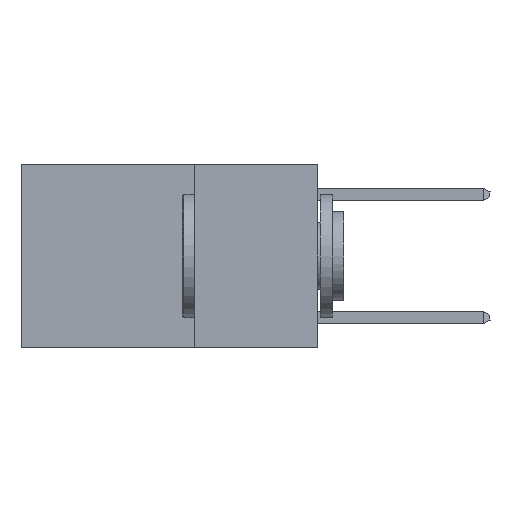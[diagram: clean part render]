
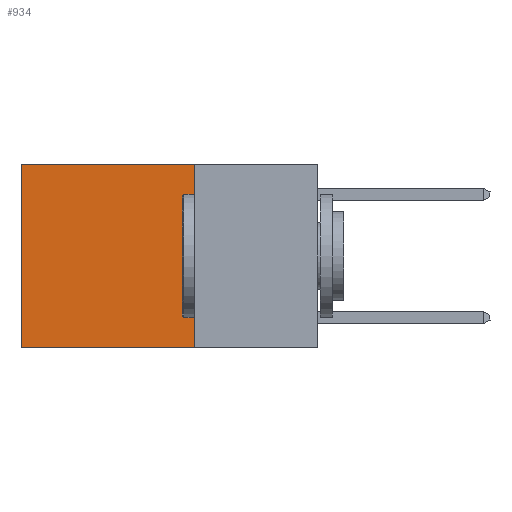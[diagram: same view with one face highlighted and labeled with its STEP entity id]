
A CAD part, left-side view. The second image highlights one B-rep face of the part: STEP entity #934.
In plain terms, the highlighted planar face has unit normal (-1, 0, 0).
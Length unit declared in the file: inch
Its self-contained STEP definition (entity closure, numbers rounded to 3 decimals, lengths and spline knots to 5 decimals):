
#934 = ADVANCED_FACE ( 'NONE', ( #4417 ), #14339, .F. ) ;
#2465 = LINE ( 'NONE', #10649, #8367 ) ;
#3136 = CARTESIAN_POINT ( 'NONE',  ( 0.2625, 0.25, 0. ) ) ;
#3146 = CARTESIAN_POINT ( 'NONE',  ( 0.2625, 0.25, -0.37 ) ) ;
#4417 = FACE_OUTER_BOUND ( 'NONE', #13851, .T. ) ;
#5045 = CARTESIAN_POINT ( 'NONE',  ( 0.2625, 0.6, 0. ) ) ;
#5541 = LINE ( 'NONE', #3146, #17997 ) ;
#6002 = CARTESIAN_POINT ( 'NONE',  ( 0.2625, 0.6, 0. ) ) ;
#6130 = AXIS2_PLACEMENT_3D ( 'NONE', #20787, #12459, #12589 ) ;
#6370 = CARTESIAN_POINT ( 'NONE',  ( 0.2625, 0.25, -0.37 ) ) ;
#8367 = VECTOR ( 'NONE', #18841, 39.37008 ) ;
#8741 = EDGE_CURVE ( 'NONE', #16602, #24817, #14041, .T. ) ;
#8846 = VECTOR ( 'NONE', #17084, 39.37008 ) ;
#9603 = VECTOR ( 'NONE', #22245, 39.37008 ) ;
#10649 = CARTESIAN_POINT ( 'NONE',  ( 0.2625, 0.25, 0. ) ) ;
#12417 = EDGE_CURVE ( 'NONE', #18968, #16602, #23252, .T. ) ;
#12459 = DIRECTION ( 'NONE',  ( 1., 0., 0. ) ) ;
#12589 = DIRECTION ( 'NONE',  ( 0., 0., -1. ) ) ;
#12799 = ORIENTED_EDGE ( 'NONE', *, *, #21337, .F. ) ;
#13851 = EDGE_LOOP ( 'NONE', ( #15248, #22645, #12799, #26347 ) ) ;
#14041 = LINE ( 'NONE', #6002, #9603 ) ;
#14339 = PLANE ( 'NONE',  #6130 ) ;
#15248 = ORIENTED_EDGE ( 'NONE', *, *, #8741, .T. ) ;
#15681 = EDGE_CURVE ( 'NONE', #16878, #24817, #5541, .T. ) ;
#16602 = VERTEX_POINT ( 'NONE', #5045 ) ;
#16878 = VERTEX_POINT ( 'NONE', #6370 ) ;
#17084 = DIRECTION ( 'NONE',  ( 0., 1., 0. ) ) ;
#17997 = VECTOR ( 'NONE', #25799, 39.37008 ) ;
#18841 = DIRECTION ( 'NONE',  ( 0., 0., -1. ) ) ;
#18968 = VERTEX_POINT ( 'NONE', #19368 ) ;
#19368 = CARTESIAN_POINT ( 'NONE',  ( 0.2625, 0.25, 0. ) ) ;
#20787 = CARTESIAN_POINT ( 'NONE',  ( 0.2625, 0.25, 0. ) ) ;
#21337 = EDGE_CURVE ( 'NONE', #18968, #16878, #2465, .T. ) ;
#22245 = DIRECTION ( 'NONE',  ( 0., 0., -1. ) ) ;
#22267 = CARTESIAN_POINT ( 'NONE',  ( 0.2625, 0.6, -0.37 ) ) ;
#22645 = ORIENTED_EDGE ( 'NONE', *, *, #15681, .F. ) ;
#23252 = LINE ( 'NONE', #3136, #8846 ) ;
#24817 = VERTEX_POINT ( 'NONE', #22267 ) ;
#25799 = DIRECTION ( 'NONE',  ( 0., 1., 0. ) ) ;
#26347 = ORIENTED_EDGE ( 'NONE', *, *, #12417, .T. ) ;
